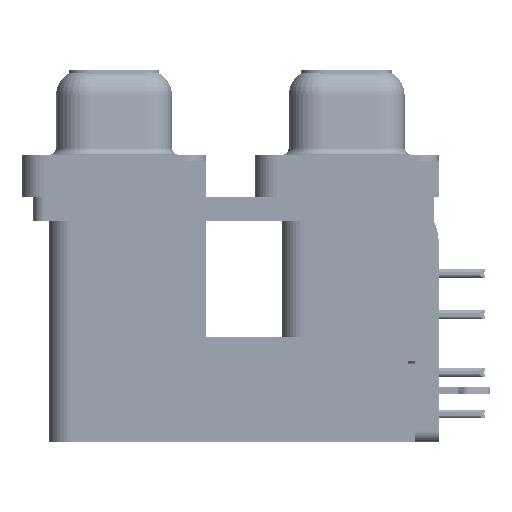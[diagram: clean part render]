
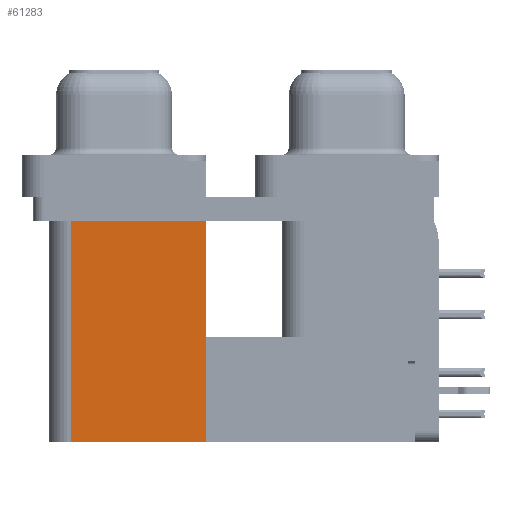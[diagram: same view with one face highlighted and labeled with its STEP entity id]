
A CAD part, left-side view. The second image highlights one B-rep face of the part: STEP entity #61283.
In plain terms, the highlighted planar face has unit normal (-1, 0, 0).
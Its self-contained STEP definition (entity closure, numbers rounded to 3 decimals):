
#2135 = LINE ( 'NONE', #59820, #40456 ) ;
#2986 = AXIS2_PLACEMENT_3D ( 'NONE', #6256, #11603, #25482 ) ;
#6068 = ORIENTED_EDGE ( 'NONE', *, *, #24304, .T. ) ;
#6256 = CARTESIAN_POINT ( 'NONE',  ( 3.7, 9.6, -19.2 ) ) ;
#9896 = VECTOR ( 'NONE', #49914, 1000. ) ;
#10237 = VERTEX_POINT ( 'NONE', #53942 ) ;
#10592 = VECTOR ( 'NONE', #39005, 1000. ) ;
#11210 = LINE ( 'NONE', #19750, #10592 ) ;
#11519 = EDGE_LOOP ( 'NONE', ( #37386, #34870, #47271, #6068 ) ) ;
#11603 = DIRECTION ( 'NONE',  ( 1., 0., 0. ) ) ;
#16893 = CARTESIAN_POINT ( 'NONE',  ( 3.7, 18.8, -2.5 ) ) ;
#19608 = EDGE_CURVE ( 'NONE', #32356, #61684, #30682, .T. ) ;
#19750 = CARTESIAN_POINT ( 'NONE',  ( 3.7, 9.6, -19.2 ) ) ;
#23229 = CARTESIAN_POINT ( 'NONE',  ( 3.7, 18.8, -19.2 ) ) ;
#24304 = EDGE_CURVE ( 'NONE', #10237, #32356, #2135, .T. ) ;
#25482 = DIRECTION ( 'NONE',  ( 0., 1., 0. ) ) ;
#29728 = CARTESIAN_POINT ( 'NONE',  ( 3.7, 9.6, -2.5 ) ) ;
#29847 = DIRECTION ( 'NONE',  ( 0., 0., 1. ) ) ;
#30682 = LINE ( 'NONE', #50232, #9896 ) ;
#32356 = VERTEX_POINT ( 'NONE', #29728 ) ;
#34870 = ORIENTED_EDGE ( 'NONE', *, *, #40726, .F. ) ;
#36228 = FACE_OUTER_BOUND ( 'NONE', #11519, .T. ) ;
#37386 = ORIENTED_EDGE ( 'NONE', *, *, #19608, .T. ) ;
#39005 = DIRECTION ( 'NONE',  ( 0., 1., 0. ) ) ;
#39726 = EDGE_CURVE ( 'NONE', #10237, #42584, #11210, .T. ) ;
#40456 = VECTOR ( 'NONE', #54487, 1000. ) ;
#40726 = EDGE_CURVE ( 'NONE', #42584, #61684, #59135, .T. ) ;
#42584 = VERTEX_POINT ( 'NONE', #23229 ) ;
#47271 = ORIENTED_EDGE ( 'NONE', *, *, #39726, .F. ) ;
#48759 = CARTESIAN_POINT ( 'NONE',  ( 3.7, 18.8, -19.2 ) ) ;
#49914 = DIRECTION ( 'NONE',  ( 0., 1., 0. ) ) ;
#50232 = CARTESIAN_POINT ( 'NONE',  ( 3.7, 9.6, -2.5 ) ) ;
#53942 = CARTESIAN_POINT ( 'NONE',  ( 3.7, 9.6, -19.2 ) ) ;
#54487 = DIRECTION ( 'NONE',  ( 0., 0., 1. ) ) ;
#54802 = PLANE ( 'NONE',  #2986 ) ;
#59135 = LINE ( 'NONE', #48759, #59946 ) ;
#59820 = CARTESIAN_POINT ( 'NONE',  ( 3.7, 9.6, -19.2 ) ) ;
#59946 = VECTOR ( 'NONE', #29847, 1000. ) ;
#61283 = ADVANCED_FACE ( 'NONE', ( #36228 ), #54802, .F. ) ;
#61684 = VERTEX_POINT ( 'NONE', #16893 ) ;
